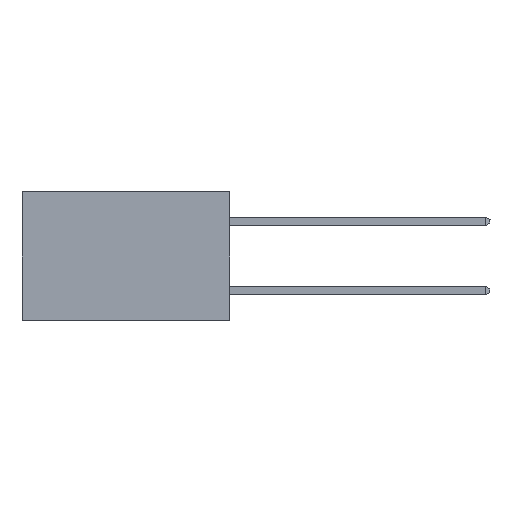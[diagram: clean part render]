
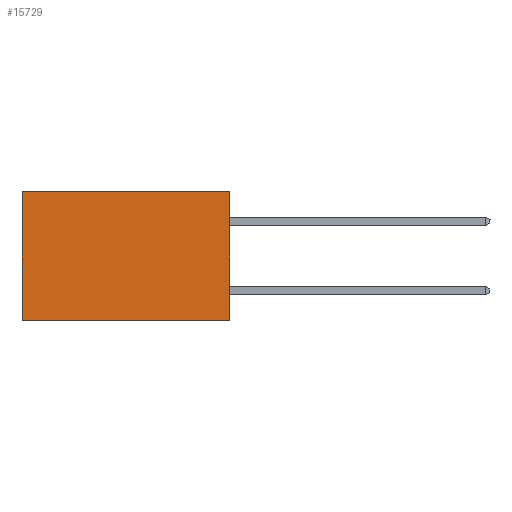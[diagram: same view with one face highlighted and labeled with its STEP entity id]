
A CAD part, left-side view. The second image highlights one B-rep face of the part: STEP entity #15729.
In plain terms, the highlighted planar face has unit normal (-1, 0, 0).
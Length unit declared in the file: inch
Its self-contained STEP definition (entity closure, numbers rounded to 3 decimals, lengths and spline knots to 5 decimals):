
#511 = VERTEX_POINT ( 'NONE', #546 ) ;
#546 = CARTESIAN_POINT ( 'NONE',  ( 0.2615, 0.6, 0. ) ) ;
#1468 = EDGE_CURVE ( 'NONE', #18679, #17755, #6604, .T. ) ;
#2045 = ORIENTED_EDGE ( 'NONE', *, *, #18864, .F. ) ;
#2678 = CARTESIAN_POINT ( 'NONE',  ( 0.2615, 0., 0. ) ) ;
#2820 = DIRECTION ( 'NONE',  ( 0., 1., 0. ) ) ;
#3114 = PLANE ( 'NONE',  #20210 ) ;
#4264 = DIRECTION ( 'NONE',  ( 0., 1., 0. ) ) ;
#4268 = EDGE_CURVE ( 'NONE', #511, #17755, #13654, .T. ) ;
#4889 = DIRECTION ( 'NONE',  ( 1., 0., 0. ) ) ;
#5527 = EDGE_CURVE ( 'NONE', #7395, #511, #20219, .T. ) ;
#6313 = DIRECTION ( 'NONE',  ( 0., 0., -1. ) ) ;
#6495 = CARTESIAN_POINT ( 'NONE',  ( 0.2615, 0.6, -0.37 ) ) ;
#6604 = LINE ( 'NONE', #21805, #19649 ) ;
#7395 = VERTEX_POINT ( 'NONE', #10235 ) ;
#8147 = VECTOR ( 'NONE', #21916, 39.37008 ) ;
#8608 = VECTOR ( 'NONE', #6313, 39.37008 ) ;
#9716 = CARTESIAN_POINT ( 'NONE',  ( 0.2615, 0., -0.37 ) ) ;
#10235 = CARTESIAN_POINT ( 'NONE',  ( 0.2615, 0., 0. ) ) ;
#11632 = CARTESIAN_POINT ( 'NONE',  ( 0.2615, 0.6, -0.37 ) ) ;
#12332 = ORIENTED_EDGE ( 'NONE', *, *, #1468, .F. ) ;
#13371 = EDGE_LOOP ( 'NONE', ( #20756, #12332, #2045, #18944 ) ) ;
#13411 = CARTESIAN_POINT ( 'NONE',  ( 0.2615, 0., -0.37 ) ) ;
#13654 = LINE ( 'NONE', #6495, #8608 ) ;
#15711 = VECTOR ( 'NONE', #2820, 39.37008 ) ;
#15729 = ADVANCED_FACE ( 'NONE', ( #19512 ), #3114, .F. ) ;
#16843 = DIRECTION ( 'NONE',  ( 0., 0., -1. ) ) ;
#17222 = LINE ( 'NONE', #20247, #8147 ) ;
#17755 = VERTEX_POINT ( 'NONE', #11632 ) ;
#18679 = VERTEX_POINT ( 'NONE', #9716 ) ;
#18864 = EDGE_CURVE ( 'NONE', #7395, #18679, #17222, .T. ) ;
#18944 = ORIENTED_EDGE ( 'NONE', *, *, #5527, .T. ) ;
#19512 = FACE_OUTER_BOUND ( 'NONE', #13371, .T. ) ;
#19649 = VECTOR ( 'NONE', #4264, 39.37008 ) ;
#20210 = AXIS2_PLACEMENT_3D ( 'NONE', #13411, #4889, #16843 ) ;
#20219 = LINE ( 'NONE', #2678, #15711 ) ;
#20247 = CARTESIAN_POINT ( 'NONE',  ( 0.2615, 0., -0.37 ) ) ;
#20756 = ORIENTED_EDGE ( 'NONE', *, *, #4268, .T. ) ;
#21805 = CARTESIAN_POINT ( 'NONE',  ( 0.2615, 0., -0.37 ) ) ;
#21916 = DIRECTION ( 'NONE',  ( 0., 0., -1. ) ) ;
